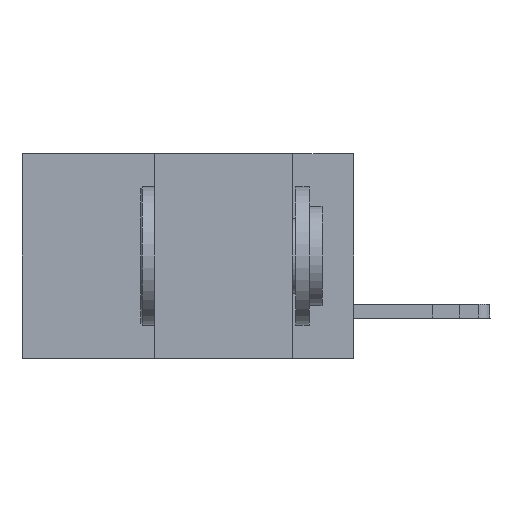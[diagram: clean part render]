
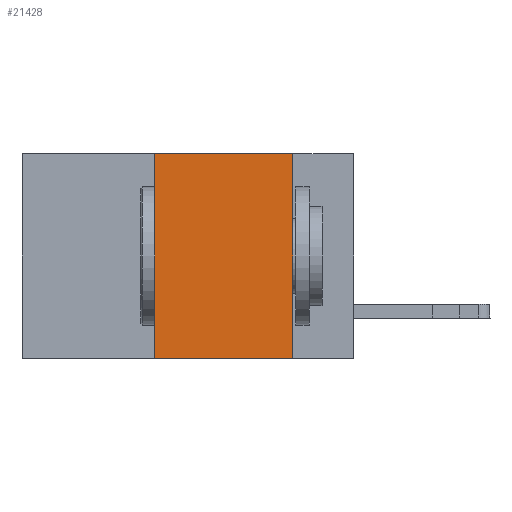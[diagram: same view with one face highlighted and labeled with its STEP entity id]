
A CAD part, left-side view. The second image highlights one B-rep face of the part: STEP entity #21428.
In plain terms, the highlighted planar face has unit normal (-1, 0, 0).
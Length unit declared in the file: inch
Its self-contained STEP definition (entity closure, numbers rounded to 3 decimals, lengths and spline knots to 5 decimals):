
#559 = EDGE_CURVE ( 'NONE', #23713, #5029, #15241, .T. ) ;
#1100 = DIRECTION ( 'NONE',  ( 1., 0., 0. ) ) ;
#1345 = FACE_OUTER_BOUND ( 'NONE', #13577, .T. ) ;
#2430 = DIRECTION ( 'NONE',  ( 0., -1., 0. ) ) ;
#3182 = ORIENTED_EDGE ( 'NONE', *, *, #18110, .T. ) ;
#4685 = LINE ( 'NONE', #15857, #15182 ) ;
#5029 = VERTEX_POINT ( 'NONE', #7749 ) ;
#5581 = ORIENTED_EDGE ( 'NONE', *, *, #9117, .F. ) ;
#6019 = DIRECTION ( 'NONE',  ( 0., -1., 0. ) ) ;
#6642 = CARTESIAN_POINT ( 'NONE',  ( 0., 0.11, -0.37 ) ) ;
#7693 = VECTOR ( 'NONE', #2430, 39.37008 ) ;
#7749 = CARTESIAN_POINT ( 'NONE',  ( 0., 0.36, 0. ) ) ;
#7987 = LINE ( 'NONE', #20792, #21436 ) ;
#9117 = EDGE_CURVE ( 'NONE', #21365, #21549, #4685, .T. ) ;
#12391 = PLANE ( 'NONE',  #19937 ) ;
#12639 = DIRECTION ( 'NONE',  ( 0., 0., -1. ) ) ;
#13577 = EDGE_LOOP ( 'NONE', ( #5581, #22827, #20197, #3182 ) ) ;
#13591 = CARTESIAN_POINT ( 'NONE',  ( 0., 0.6, 0. ) ) ;
#13625 = CARTESIAN_POINT ( 'NONE',  ( 0., 0.36, 0. ) ) ;
#15182 = VECTOR ( 'NONE', #12639, 39.37008 ) ;
#15241 = LINE ( 'NONE', #13625, #18805 ) ;
#15857 = CARTESIAN_POINT ( 'NONE',  ( 0., 0.11, 0. ) ) ;
#16620 = DIRECTION ( 'NONE',  ( 0., 0., 1. ) ) ;
#17703 = CARTESIAN_POINT ( 'NONE',  ( 0., 0.6, 0. ) ) ;
#18110 = EDGE_CURVE ( 'NONE', #23713, #21549, #7987, .T. ) ;
#18563 = EDGE_CURVE ( 'NONE', #5029, #21365, #20757, .T. ) ;
#18805 = VECTOR ( 'NONE', #16620, 39.37008 ) ;
#19786 = DIRECTION ( 'NONE',  ( 0., 0., -1. ) ) ;
#19937 = AXIS2_PLACEMENT_3D ( 'NONE', #17703, #1100, #19786 ) ;
#20197 = ORIENTED_EDGE ( 'NONE', *, *, #559, .F. ) ;
#20576 = CARTESIAN_POINT ( 'NONE',  ( 0., 0.11, 0. ) ) ;
#20586 = CARTESIAN_POINT ( 'NONE',  ( 0., 0.36, -0.37 ) ) ;
#20757 = LINE ( 'NONE', #13591, #7693 ) ;
#20792 = CARTESIAN_POINT ( 'NONE',  ( 0., 0.6, -0.37 ) ) ;
#21365 = VERTEX_POINT ( 'NONE', #20576 ) ;
#21428 = ADVANCED_FACE ( 'NONE', ( #1345 ), #12391, .F. ) ;
#21436 = VECTOR ( 'NONE', #6019, 39.37008 ) ;
#21549 = VERTEX_POINT ( 'NONE', #6642 ) ;
#22827 = ORIENTED_EDGE ( 'NONE', *, *, #18563, .F. ) ;
#23713 = VERTEX_POINT ( 'NONE', #20586 ) ;
